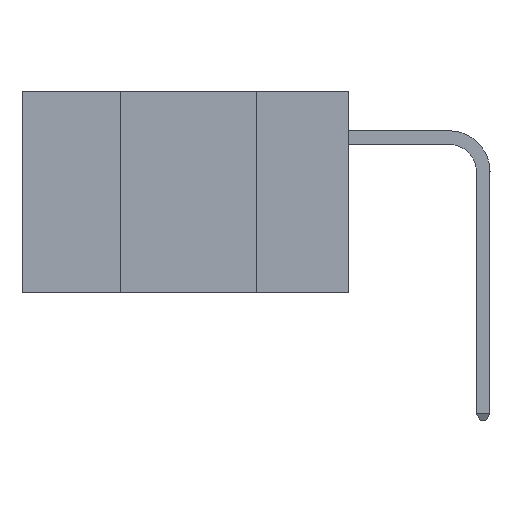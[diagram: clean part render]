
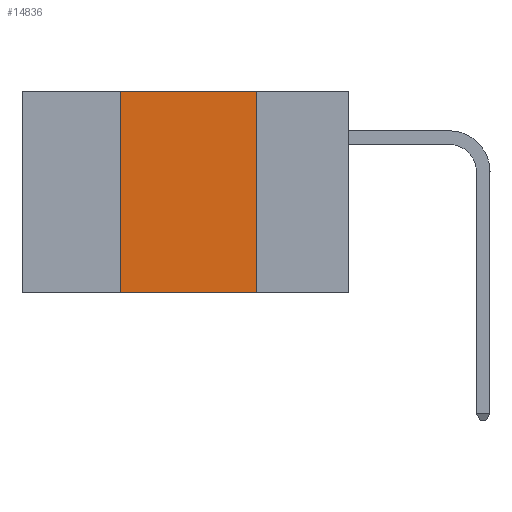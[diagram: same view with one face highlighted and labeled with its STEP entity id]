
A CAD part, left-side view. The second image highlights one B-rep face of the part: STEP entity #14836.
In plain terms, the highlighted planar face has unit normal (-1, 0, 0).
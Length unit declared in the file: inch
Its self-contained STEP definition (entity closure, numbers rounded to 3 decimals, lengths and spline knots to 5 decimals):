
#474 = EDGE_CURVE ( 'NONE', #10563, #6768, #8845, .T. ) ;
#790 = PLANE ( 'NONE',  #3351 ) ;
#1174 = VERTEX_POINT ( 'NONE', #3380 ) ;
#1771 = VECTOR ( 'NONE', #3227, 39.37008 ) ;
#2049 = DIRECTION ( 'NONE',  ( 0., 0., -1. ) ) ;
#2723 = VECTOR ( 'NONE', #3039, 39.37008 ) ;
#3030 = DIRECTION ( 'NONE',  ( 0., 0., 1. ) ) ;
#3039 = DIRECTION ( 'NONE',  ( 0., 0., -1. ) ) ;
#3124 = ORIENTED_EDGE ( 'NONE', *, *, #474, .F. ) ;
#3169 = ORIENTED_EDGE ( 'NONE', *, *, #11296, .F. ) ;
#3198 = ORIENTED_EDGE ( 'NONE', *, *, #14056, .F. ) ;
#3216 = ORIENTED_EDGE ( 'NONE', *, *, #12523, .T. ) ;
#3227 = DIRECTION ( 'NONE',  ( 0., -1., 0. ) ) ;
#3351 = AXIS2_PLACEMENT_3D ( 'NONE', #5610, #8986, #2049 ) ;
#3380 = CARTESIAN_POINT ( 'NONE',  ( 0., 0.42, 0. ) ) ;
#3687 = FACE_OUTER_BOUND ( 'NONE', #12684, .T. ) ;
#4269 = CARTESIAN_POINT ( 'NONE',  ( 0., 0.17, 0. ) ) ;
#4890 = VERTEX_POINT ( 'NONE', #14901 ) ;
#5610 = CARTESIAN_POINT ( 'NONE',  ( 0., 0.6, 0. ) ) ;
#5677 = CARTESIAN_POINT ( 'NONE',  ( 0., 0.6, -0.37 ) ) ;
#6286 = CARTESIAN_POINT ( 'NONE',  ( 0., 0.17, -0.37 ) ) ;
#6719 = CARTESIAN_POINT ( 'NONE',  ( 0., 0.6, 0. ) ) ;
#6768 = VERTEX_POINT ( 'NONE', #6286 ) ;
#6787 = DIRECTION ( 'NONE',  ( 0., -1., 0. ) ) ;
#6961 = VECTOR ( 'NONE', #6787, 39.37008 ) ;
#7970 = LINE ( 'NONE', #6719, #1771 ) ;
#8542 = CARTESIAN_POINT ( 'NONE',  ( 0., 0.17, 0. ) ) ;
#8748 = CARTESIAN_POINT ( 'NONE',  ( 0., 0.42, 0. ) ) ;
#8845 = LINE ( 'NONE', #8542, #2723 ) ;
#8986 = DIRECTION ( 'NONE',  ( 1., 0., 0. ) ) ;
#9394 = VECTOR ( 'NONE', #3030, 39.37008 ) ;
#9745 = LINE ( 'NONE', #8748, #9394 ) ;
#9979 = LINE ( 'NONE', #5677, #6961 ) ;
#10563 = VERTEX_POINT ( 'NONE', #4269 ) ;
#11296 = EDGE_CURVE ( 'NONE', #1174, #10563, #7970, .T. ) ;
#12523 = EDGE_CURVE ( 'NONE', #4890, #6768, #9979, .T. ) ;
#12684 = EDGE_LOOP ( 'NONE', ( #3124, #3169, #3198, #3216 ) ) ;
#14056 = EDGE_CURVE ( 'NONE', #4890, #1174, #9745, .T. ) ;
#14836 = ADVANCED_FACE ( 'NONE', ( #3687 ), #790, .F. ) ;
#14901 = CARTESIAN_POINT ( 'NONE',  ( 0., 0.42, -0.37 ) ) ;
